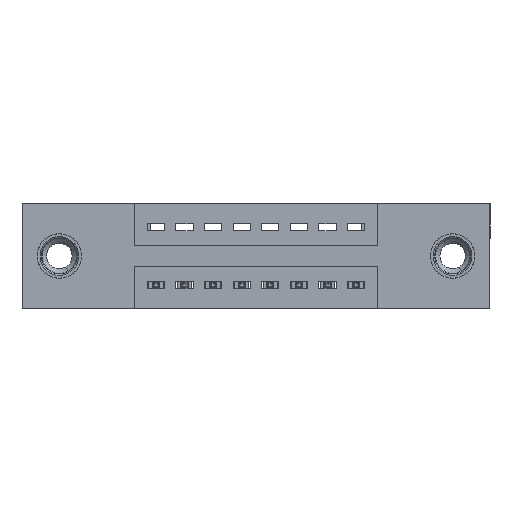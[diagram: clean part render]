
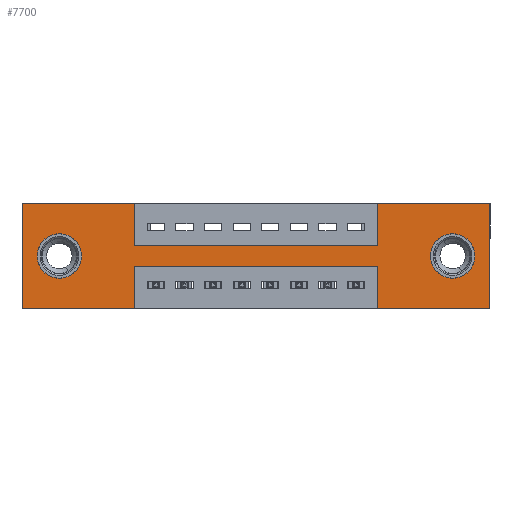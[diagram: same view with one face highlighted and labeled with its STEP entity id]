
A CAD part, front view. The second image highlights one B-rep face of the part: STEP entity #7700.
In plain terms, the highlighted planar face has unit normal (0, -1, 0).
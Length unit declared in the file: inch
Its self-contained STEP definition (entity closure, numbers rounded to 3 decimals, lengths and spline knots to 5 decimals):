
#7 = CIRCLE ( 'NONE', #13919, 0.078 ) ;
#260 = DIRECTION ( 'NONE',  ( 1., 0., 0. ) ) ;
#344 = CARTESIAN_POINT ( 'NONE',  ( 0.13, 0., -0.107 ) ) ;
#443 = CARTESIAN_POINT ( 'NONE',  ( 0.13, 0., -0.185 ) ) ;
#537 = ORIENTED_EDGE ( 'NONE', *, *, #7652, .T. ) ;
#539 = ORIENTED_EDGE ( 'NONE', *, *, #7005, .F. ) ;
#549 = DIRECTION ( 'NONE',  ( 0., 1., 0. ) ) ;
#655 = CARTESIAN_POINT ( 'NONE',  ( 1.635, 0., 0. ) ) ;
#663 = VERTEX_POINT ( 'NONE', #2406 ) ;
#667 = DIRECTION ( 'NONE',  ( 0., 1., 0. ) ) ;
#1254 = CARTESIAN_POINT ( 'NONE',  ( 0.3925, 0., -0.22 ) ) ;
#1401 = VECTOR ( 'NONE', #3649, 39.37008 ) ;
#1431 = EDGE_CURVE ( 'NONE', #7717, #6684, #11309, .T. ) ;
#1483 = CARTESIAN_POINT ( 'NONE',  ( 1.2425, 0., -0.37 ) ) ;
#1499 = VERTEX_POINT ( 'NONE', #2129 ) ;
#1547 = CARTESIAN_POINT ( 'NONE',  ( 1.635, 0., 0. ) ) ;
#1717 = ORIENTED_EDGE ( 'NONE', *, *, #8536, .F. ) ;
#1811 = EDGE_CURVE ( 'NONE', #12518, #8298, #2398, .T. ) ;
#1896 = FACE_OUTER_BOUND ( 'NONE', #6526, .T. ) ;
#1946 = DIRECTION ( 'NONE',  ( 0., 0., 1. ) ) ;
#1956 = LINE ( 'NONE', #13110, #10526 ) ;
#1965 = VERTEX_POINT ( 'NONE', #344 ) ;
#2129 = CARTESIAN_POINT ( 'NONE',  ( 1.2425, 0., -0.15 ) ) ;
#2261 = CARTESIAN_POINT ( 'NONE',  ( 0., 0., 0. ) ) ;
#2376 = CIRCLE ( 'NONE', #4709, 0.078 ) ;
#2397 = CARTESIAN_POINT ( 'NONE',  ( 0., 0., 0. ) ) ;
#2398 = LINE ( 'NONE', #14741, #15099 ) ;
#2406 = CARTESIAN_POINT ( 'NONE',  ( 0., 0., -0.37 ) ) ;
#2574 = CARTESIAN_POINT ( 'NONE',  ( 1.2425, 0., -0.22 ) ) ;
#2605 = DIRECTION ( 'NONE',  ( 0., 0., 1. ) ) ;
#2636 = LINE ( 'NONE', #9582, #14946 ) ;
#2928 = DIRECTION ( 'NONE',  ( 0., 0., 1. ) ) ;
#2959 = ORIENTED_EDGE ( 'NONE', *, *, #3027, .F. ) ;
#3027 = EDGE_CURVE ( 'NONE', #1499, #7717, #8531, .T. ) ;
#3085 = LINE ( 'NONE', #7389, #10966 ) ;
#3223 = VECTOR ( 'NONE', #10884, 39.37008 ) ;
#3289 = EDGE_LOOP ( 'NONE', ( #537, #6931 ) ) ;
#3297 = DIRECTION ( 'NONE',  ( 1., 0., 0. ) ) ;
#3649 = DIRECTION ( 'NONE',  ( 1., 0., 0. ) ) ;
#3827 = VECTOR ( 'NONE', #3297, 39.37008 ) ;
#3904 = CARTESIAN_POINT ( 'NONE',  ( 0.3925, 0., 0. ) ) ;
#4274 = EDGE_CURVE ( 'NONE', #12096, #1499, #8113, .T. ) ;
#4502 = FACE_BOUND ( 'NONE', #10698, .T. ) ;
#4557 = VERTEX_POINT ( 'NONE', #2397 ) ;
#4709 = AXIS2_PLACEMENT_3D ( 'NONE', #13634, #6529, #11181 ) ;
#4834 = EDGE_CURVE ( 'NONE', #15351, #5489, #15376, .T. ) ;
#4921 = EDGE_CURVE ( 'NONE', #6684, #12518, #13157, .T. ) ;
#5251 = CARTESIAN_POINT ( 'NONE',  ( 1.505, 0., -0.107 ) ) ;
#5449 = LINE ( 'NONE', #6304, #13312 ) ;
#5489 = VERTEX_POINT ( 'NONE', #5251 ) ;
#5868 = VECTOR ( 'NONE', #11023, 39.37008 ) ;
#5947 = ORIENTED_EDGE ( 'NONE', *, *, #4274, .F. ) ;
#6304 = CARTESIAN_POINT ( 'NONE',  ( 1.2425, 0., -0.37 ) ) ;
#6323 = CARTESIAN_POINT ( 'NONE',  ( 1.505, 0., -0.263 ) ) ;
#6526 = EDGE_LOOP ( 'NONE', ( #7691, #14930, #539, #7561, #13763, #15444, #2959, #5947, #8067, #10102, #1717, #7850 ) ) ;
#6529 = DIRECTION ( 'NONE',  ( 0., 1., 0. ) ) ;
#6684 = VERTEX_POINT ( 'NONE', #655 ) ;
#6756 = VECTOR ( 'NONE', #7361, 39.37008 ) ;
#6931 = ORIENTED_EDGE ( 'NONE', *, *, #12514, .T. ) ;
#7005 = EDGE_CURVE ( 'NONE', #8298, #15403, #5449, .T. ) ;
#7164 = DIRECTION ( 'NONE',  ( -1., 0., 0. ) ) ;
#7361 = DIRECTION ( 'NONE',  ( -1., 0., 0. ) ) ;
#7389 = CARTESIAN_POINT ( 'NONE',  ( 0., 0., 0. ) ) ;
#7414 = CARTESIAN_POINT ( 'NONE',  ( 0.3925, 0., -0.22 ) ) ;
#7561 = ORIENTED_EDGE ( 'NONE', *, *, #1811, .F. ) ;
#7652 = EDGE_CURVE ( 'NONE', #1965, #12427, #14042, .T. ) ;
#7691 = ORIENTED_EDGE ( 'NONE', *, *, #7854, .F. ) ;
#7700 = ADVANCED_FACE ( 'NONE', ( #4502, #10872, #1896 ), #11541, .T. ) ;
#7717 = VERTEX_POINT ( 'NONE', #11749 ) ;
#7850 = ORIENTED_EDGE ( 'NONE', *, *, #10135, .F. ) ;
#7854 = EDGE_CURVE ( 'NONE', #14242, #8816, #2636, .T. ) ;
#7989 = EDGE_CURVE ( 'NONE', #15403, #14242, #12722, .T. ) ;
#8067 = ORIENTED_EDGE ( 'NONE', *, *, #15368, .F. ) ;
#8113 = LINE ( 'NONE', #15342, #3827 ) ;
#8298 = VERTEX_POINT ( 'NONE', #1483 ) ;
#8531 = LINE ( 'NONE', #9115, #13973 ) ;
#8536 = EDGE_CURVE ( 'NONE', #663, #4557, #13903, .T. ) ;
#8816 = VERTEX_POINT ( 'NONE', #11823 ) ;
#9044 = CARTESIAN_POINT ( 'NONE',  ( 1.505, 0., -0.185 ) ) ;
#9115 = CARTESIAN_POINT ( 'NONE',  ( 1.2425, 0., 0. ) ) ;
#9397 = LINE ( 'NONE', #3904, #3223 ) ;
#9582 = CARTESIAN_POINT ( 'NONE',  ( 0.3925, 0., -0.37 ) ) ;
#10102 = ORIENTED_EDGE ( 'NONE', *, *, #14809, .F. ) ;
#10135 = EDGE_CURVE ( 'NONE', #8816, #663, #1956, .T. ) ;
#10280 = CARTESIAN_POINT ( 'NONE',  ( 0.13, 0., -0.185 ) ) ;
#10376 = DIRECTION ( 'NONE',  ( 0., 0., 1. ) ) ;
#10518 = CARTESIAN_POINT ( 'NONE',  ( 0.3925, 0., -0.15 ) ) ;
#10526 = VECTOR ( 'NONE', #7164, 39.37008 ) ;
#10631 = DIRECTION ( 'NONE',  ( 0., 0., -1. ) ) ;
#10698 = EDGE_LOOP ( 'NONE', ( #12397, #11986 ) ) ;
#10872 = FACE_BOUND ( 'NONE', #3289, .T. ) ;
#10884 = DIRECTION ( 'NONE',  ( 0., 0., -1. ) ) ;
#10966 = VECTOR ( 'NONE', #260, 39.37008 ) ;
#11023 = DIRECTION ( 'NONE',  ( 0., 0., -1. ) ) ;
#11181 = DIRECTION ( 'NONE',  ( 0., 0., -1. ) ) ;
#11305 = CARTESIAN_POINT ( 'NONE',  ( 1.635, 0., -0.37 ) ) ;
#11309 = LINE ( 'NONE', #11779, #1401 ) ;
#11535 = DIRECTION ( 'NONE',  ( 0., 1., 0. ) ) ;
#11541 = PLANE ( 'NONE',  #13566 ) ;
#11645 = DIRECTION ( 'NONE',  ( 0., -1., 0. ) ) ;
#11749 = CARTESIAN_POINT ( 'NONE',  ( 1.2425, 0., 0. ) ) ;
#11779 = CARTESIAN_POINT ( 'NONE',  ( 0., 0., 0. ) ) ;
#11788 = DIRECTION ( 'NONE',  ( 0., 0., 1. ) ) ;
#11823 = CARTESIAN_POINT ( 'NONE',  ( 0.3925, 0., -0.37 ) ) ;
#11986 = ORIENTED_EDGE ( 'NONE', *, *, #4834, .T. ) ;
#12070 = AXIS2_PLACEMENT_3D ( 'NONE', #10280, #667, #10376 ) ;
#12096 = VERTEX_POINT ( 'NONE', #10518 ) ;
#12397 = ORIENTED_EDGE ( 'NONE', *, *, #13937, .T. ) ;
#12427 = VERTEX_POINT ( 'NONE', #14780 ) ;
#12514 = EDGE_CURVE ( 'NONE', #12427, #1965, #7, .T. ) ;
#12518 = VERTEX_POINT ( 'NONE', #11305 ) ;
#12722 = LINE ( 'NONE', #7414, #6756 ) ;
#12877 = DIRECTION ( 'NONE',  ( 0., 0., -1. ) ) ;
#12984 = CARTESIAN_POINT ( 'NONE',  ( 0., 0., -0.37 ) ) ;
#13110 = CARTESIAN_POINT ( 'NONE',  ( 0., 0., -0.37 ) ) ;
#13157 = LINE ( 'NONE', #1547, #5868 ) ;
#13158 = VERTEX_POINT ( 'NONE', #15400 ) ;
#13253 = DIRECTION ( 'NONE',  ( 0., 0., -1. ) ) ;
#13312 = VECTOR ( 'NONE', #2605, 39.37008 ) ;
#13566 = AXIS2_PLACEMENT_3D ( 'NONE', #12984, #11645, #10631 ) ;
#13634 = CARTESIAN_POINT ( 'NONE',  ( 1.505, 0., -0.185 ) ) ;
#13638 = AXIS2_PLACEMENT_3D ( 'NONE', #9044, #11535, #12877 ) ;
#13763 = ORIENTED_EDGE ( 'NONE', *, *, #4921, .F. ) ;
#13903 = LINE ( 'NONE', #2261, #14087 ) ;
#13919 = AXIS2_PLACEMENT_3D ( 'NONE', #443, #549, #2928 ) ;
#13937 = EDGE_CURVE ( 'NONE', #5489, #15351, #2376, .T. ) ;
#13973 = VECTOR ( 'NONE', #1946, 39.37008 ) ;
#14042 = CIRCLE ( 'NONE', #12070, 0.078 ) ;
#14087 = VECTOR ( 'NONE', #11788, 39.37008 ) ;
#14242 = VERTEX_POINT ( 'NONE', #1254 ) ;
#14741 = CARTESIAN_POINT ( 'NONE',  ( 0., 0., -0.37 ) ) ;
#14780 = CARTESIAN_POINT ( 'NONE',  ( 0.13, 0., -0.263 ) ) ;
#14794 = DIRECTION ( 'NONE',  ( -1., 0., 0. ) ) ;
#14809 = EDGE_CURVE ( 'NONE', #4557, #13158, #3085, .T. ) ;
#14930 = ORIENTED_EDGE ( 'NONE', *, *, #7989, .F. ) ;
#14946 = VECTOR ( 'NONE', #13253, 39.37008 ) ;
#15099 = VECTOR ( 'NONE', #14794, 39.37008 ) ;
#15342 = CARTESIAN_POINT ( 'NONE',  ( 0.3925, 0., -0.15 ) ) ;
#15351 = VERTEX_POINT ( 'NONE', #6323 ) ;
#15368 = EDGE_CURVE ( 'NONE', #13158, #12096, #9397, .T. ) ;
#15376 = CIRCLE ( 'NONE', #13638, 0.078 ) ;
#15400 = CARTESIAN_POINT ( 'NONE',  ( 0.3925, 0., 0. ) ) ;
#15403 = VERTEX_POINT ( 'NONE', #2574 ) ;
#15444 = ORIENTED_EDGE ( 'NONE', *, *, #1431, .F. ) ;
